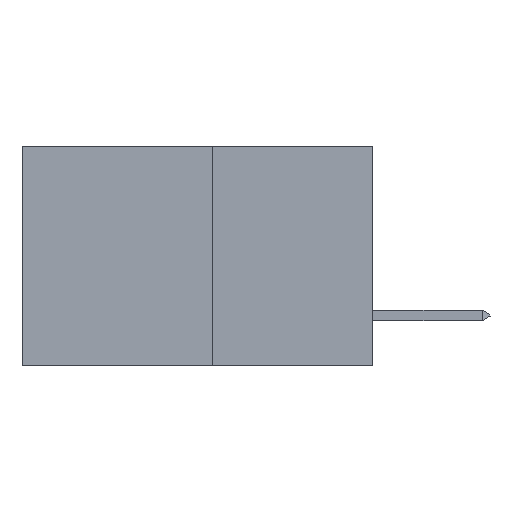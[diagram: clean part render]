
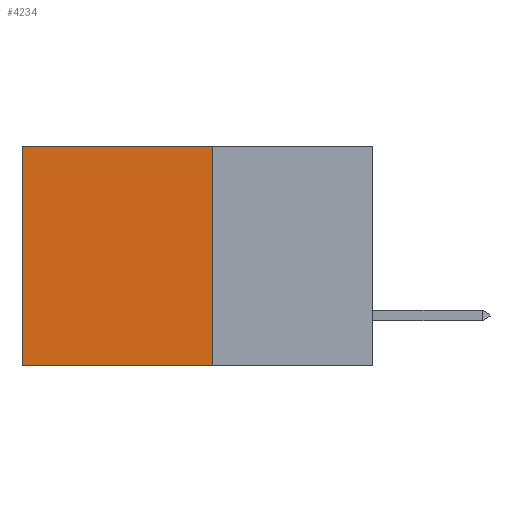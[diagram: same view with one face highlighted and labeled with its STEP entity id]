
A CAD part, left-side view. The second image highlights one B-rep face of the part: STEP entity #4234.
In plain terms, the highlighted planar face has unit normal (-1, 0, 0).
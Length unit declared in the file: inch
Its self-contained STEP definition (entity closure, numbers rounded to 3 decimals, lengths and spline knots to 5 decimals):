
#300 = DIRECTION ( 'NONE',  ( 0., 0., -1. ) ) ;
#543 = VERTEX_POINT ( 'NONE', #10203 ) ;
#593 = CARTESIAN_POINT ( 'NONE',  ( 0.277, 0.27, -0.37 ) ) ;
#753 = ORIENTED_EDGE ( 'NONE', *, *, #16507, .T. ) ;
#2138 = EDGE_LOOP ( 'NONE', ( #753, #10091, #6006, #16296 ) ) ;
#2342 = CARTESIAN_POINT ( 'NONE',  ( 0.277, 0.59, -0.37 ) ) ;
#3078 = VECTOR ( 'NONE', #15246, 39.37008 ) ;
#3237 = CARTESIAN_POINT ( 'NONE',  ( 0.277, 0.27, 0. ) ) ;
#3633 = PLANE ( 'NONE',  #12080 ) ;
#3652 = CARTESIAN_POINT ( 'NONE',  ( 0.277, 0.27, -0.37 ) ) ;
#4234 = ADVANCED_FACE ( 'NONE', ( #6001 ), #3633, .F. ) ;
#6001 = FACE_OUTER_BOUND ( 'NONE', #2138, .T. ) ;
#6006 = ORIENTED_EDGE ( 'NONE', *, *, #7086, .F. ) ;
#6210 = DIRECTION ( 'NONE',  ( 0., 1., 0. ) ) ;
#6281 = DIRECTION ( 'NONE',  ( 0., 0., -1. ) ) ;
#6347 = DIRECTION ( 'NONE',  ( 1., 0., 0. ) ) ;
#7086 = EDGE_CURVE ( 'NONE', #14993, #10880, #15745, .T. ) ;
#7456 = EDGE_CURVE ( 'NONE', #10880, #10105, #9668, .T. ) ;
#7616 = VECTOR ( 'NONE', #9638, 39.37008 ) ;
#9036 = CARTESIAN_POINT ( 'NONE',  ( 0.277, 0.27, -0.37 ) ) ;
#9638 = DIRECTION ( 'NONE',  ( 0., 1., 0. ) ) ;
#9668 = LINE ( 'NONE', #3652, #13147 ) ;
#10001 = CARTESIAN_POINT ( 'NONE',  ( 0.277, 0.59, -0.37 ) ) ;
#10091 = ORIENTED_EDGE ( 'NONE', *, *, #7456, .F. ) ;
#10105 = VERTEX_POINT ( 'NONE', #10001 ) ;
#10203 = CARTESIAN_POINT ( 'NONE',  ( 0.277, 0.59, 0. ) ) ;
#10500 = EDGE_CURVE ( 'NONE', #14993, #543, #14848, .T. ) ;
#10880 = VERTEX_POINT ( 'NONE', #9036 ) ;
#11948 = VECTOR ( 'NONE', #300, 39.37008 ) ;
#12080 = AXIS2_PLACEMENT_3D ( 'NONE', #14381, #6347, #6281 ) ;
#13147 = VECTOR ( 'NONE', #6210, 39.37008 ) ;
#13528 = CARTESIAN_POINT ( 'NONE',  ( 0.277, 0.27, 0. ) ) ;
#14381 = CARTESIAN_POINT ( 'NONE',  ( 0.277, 0.27, -0.37 ) ) ;
#14848 = LINE ( 'NONE', #13528, #7616 ) ;
#14993 = VERTEX_POINT ( 'NONE', #3237 ) ;
#15246 = DIRECTION ( 'NONE',  ( 0., 0., -1. ) ) ;
#15745 = LINE ( 'NONE', #593, #11948 ) ;
#15936 = LINE ( 'NONE', #2342, #3078 ) ;
#16296 = ORIENTED_EDGE ( 'NONE', *, *, #10500, .T. ) ;
#16507 = EDGE_CURVE ( 'NONE', #543, #10105, #15936, .T. ) ;
